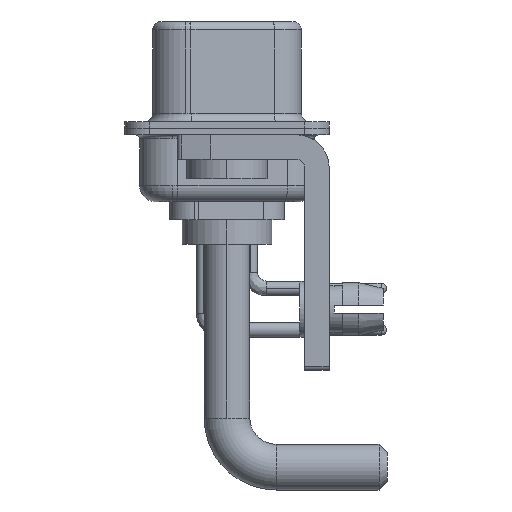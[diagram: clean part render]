
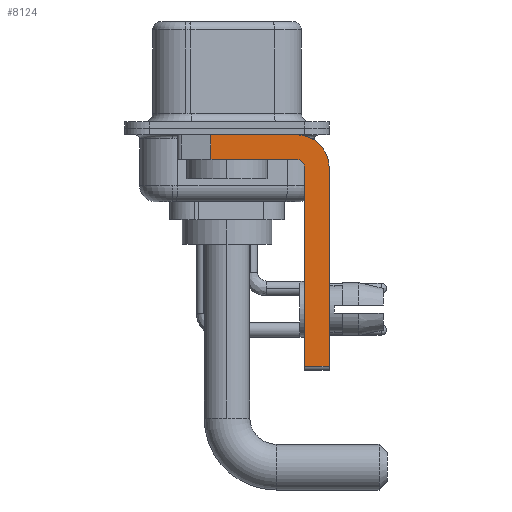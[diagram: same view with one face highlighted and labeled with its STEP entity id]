
A CAD part, left-side view. The second image highlights one B-rep face of the part: STEP entity #8124.
In plain terms, the highlighted planar face has unit normal (-1, 0, 0).
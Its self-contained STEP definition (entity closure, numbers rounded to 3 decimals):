
#136 = DIRECTION ( 'NONE',  ( -1., 0., 0. ) ) ;
#434 = VERTEX_POINT ( 'NONE', #14477 ) ;
#1274 = VECTOR ( 'NONE', #3018, 1000. ) ;
#1788 = FACE_OUTER_BOUND ( 'NONE', #2938, .T. ) ;
#2938 = EDGE_LOOP ( 'NONE', ( #14856, #8297, #17866, #10923, #26961, #12679, #23929, #24314 ) ) ;
#3018 = DIRECTION ( 'NONE',  ( 0., 1., 0. ) ) ;
#3985 = LINE ( 'NONE', #7838, #6284 ) ;
#4906 = VERTEX_POINT ( 'NONE', #17420 ) ;
#5305 = EDGE_CURVE ( 'NONE', #26035, #11525, #15203, .T. ) ;
#5497 = VERTEX_POINT ( 'NONE', #5539 ) ;
#5539 = CARTESIAN_POINT ( 'NONE',  ( -2.9, -4.75, -2.4 ) ) ;
#6021 = CIRCLE ( 'NONE', #24782, 2. ) ;
#6191 = VECTOR ( 'NONE', #12241, 1000. ) ;
#6235 = LINE ( 'NONE', #12524, #6191 ) ;
#6284 = VECTOR ( 'NONE', #20522, 1000. ) ;
#6534 = VERTEX_POINT ( 'NONE', #12805 ) ;
#7108 = VECTOR ( 'NONE', #8294, 1000. ) ;
#7243 = LINE ( 'NONE', #9422, #9739 ) ;
#7838 = CARTESIAN_POINT ( 'NONE',  ( -2.9, 3., -0.4 ) ) ;
#8124 = ADVANCED_FACE ( 'NONE', ( #1788 ), #10129, .F. ) ;
#8294 = DIRECTION ( 'NONE',  ( 0., 0., -1. ) ) ;
#8297 = ORIENTED_EDGE ( 'NONE', *, *, #20016, .T. ) ;
#8485 = DIRECTION ( 'NONE',  ( 0., 0., 1. ) ) ;
#9416 = AXIS2_PLACEMENT_3D ( 'NONE', #13697, #22038, #11648 ) ;
#9422 = CARTESIAN_POINT ( 'NONE',  ( -2.9, -4.75, -14.8 ) ) ;
#9739 = VECTOR ( 'NONE', #13112, 1000. ) ;
#10129 = PLANE ( 'NONE',  #9416 ) ;
#10383 = EDGE_CURVE ( 'NONE', #18088, #6534, #6021, .T. ) ;
#10923 = ORIENTED_EDGE ( 'NONE', *, *, #11532, .F. ) ;
#11525 = VERTEX_POINT ( 'NONE', #13116 ) ;
#11532 = EDGE_CURVE ( 'NONE', #5497, #26035, #26514, .T. ) ;
#11648 = DIRECTION ( 'NONE',  ( 0., 0., -1. ) ) ;
#12241 = DIRECTION ( 'NONE',  ( 0., -1., 0. ) ) ;
#12322 = CARTESIAN_POINT ( 'NONE',  ( -2.9, -4.25, -0.4 ) ) ;
#12524 = CARTESIAN_POINT ( 'NONE',  ( -2.9, -4.25, -14.55 ) ) ;
#12679 = ORIENTED_EDGE ( 'NONE', *, *, #15913, .T. ) ;
#12805 = CARTESIAN_POINT ( 'NONE',  ( -2.9, -6.25, -2.4 ) ) ;
#13112 = DIRECTION ( 'NONE',  ( 0., 0., 1. ) ) ;
#13116 = CARTESIAN_POINT ( 'NONE',  ( -2.9, 0.978, -1.9 ) ) ;
#13400 = CARTESIAN_POINT ( 'NONE',  ( -2.9, -4.25, -1.9 ) ) ;
#13697 = CARTESIAN_POINT ( 'NONE',  ( -2.9, -4.25, -2.4 ) ) ;
#14184 = DIRECTION ( 'NONE',  ( 1., 0., 0. ) ) ;
#14197 = CARTESIAN_POINT ( 'NONE',  ( -2.9, -4.25, -1.9 ) ) ;
#14477 = CARTESIAN_POINT ( 'NONE',  ( -2.9, 0.978, -0.4 ) ) ;
#14613 = DIRECTION ( 'NONE',  ( 0., 0., -1. ) ) ;
#14856 = ORIENTED_EDGE ( 'NONE', *, *, #19438, .F. ) ;
#15203 = LINE ( 'NONE', #13400, #1274 ) ;
#15913 = EDGE_CURVE ( 'NONE', #4906, #18030, #6235, .T. ) ;
#16151 = CARTESIAN_POINT ( 'NONE',  ( -2.9, -6.25, -14.55 ) ) ;
#16938 = LINE ( 'NONE', #17212, #18801 ) ;
#17212 = CARTESIAN_POINT ( 'NONE',  ( -2.9, 0.978, -1.9 ) ) ;
#17420 = CARTESIAN_POINT ( 'NONE',  ( -2.9, -4.75, -14.55 ) ) ;
#17866 = ORIENTED_EDGE ( 'NONE', *, *, #5305, .F. ) ;
#18030 = VERTEX_POINT ( 'NONE', #16151 ) ;
#18088 = VERTEX_POINT ( 'NONE', #12322 ) ;
#18156 = DIRECTION ( 'NONE',  ( 0., 0., -1. ) ) ;
#18420 = CARTESIAN_POINT ( 'NONE',  ( -2.9, -4.25, -2.4 ) ) ;
#18543 = EDGE_CURVE ( 'NONE', #6534, #18030, #20996, .T. ) ;
#18683 = CARTESIAN_POINT ( 'NONE',  ( -2.9, -6.25, -2.4 ) ) ;
#18801 = VECTOR ( 'NONE', #14613, 1000. ) ;
#19438 = EDGE_CURVE ( 'NONE', #434, #18088, #3985, .T. ) ;
#20016 = EDGE_CURVE ( 'NONE', #434, #11525, #16938, .T. ) ;
#20522 = DIRECTION ( 'NONE',  ( 0., -1., 0. ) ) ;
#20996 = LINE ( 'NONE', #18683, #7108 ) ;
#22038 = DIRECTION ( 'NONE',  ( 1., 0., 0. ) ) ;
#22131 = AXIS2_PLACEMENT_3D ( 'NONE', #22967, #136, #8485 ) ;
#22774 = EDGE_CURVE ( 'NONE', #4906, #5497, #7243, .T. ) ;
#22967 = CARTESIAN_POINT ( 'NONE',  ( -2.9, -4.25, -2.4 ) ) ;
#23929 = ORIENTED_EDGE ( 'NONE', *, *, #18543, .F. ) ;
#24314 = ORIENTED_EDGE ( 'NONE', *, *, #10383, .F. ) ;
#24782 = AXIS2_PLACEMENT_3D ( 'NONE', #18420, #14184, #18156 ) ;
#26035 = VERTEX_POINT ( 'NONE', #14197 ) ;
#26514 = CIRCLE ( 'NONE', #22131, 0.5 ) ;
#26961 = ORIENTED_EDGE ( 'NONE', *, *, #22774, .F. ) ;
